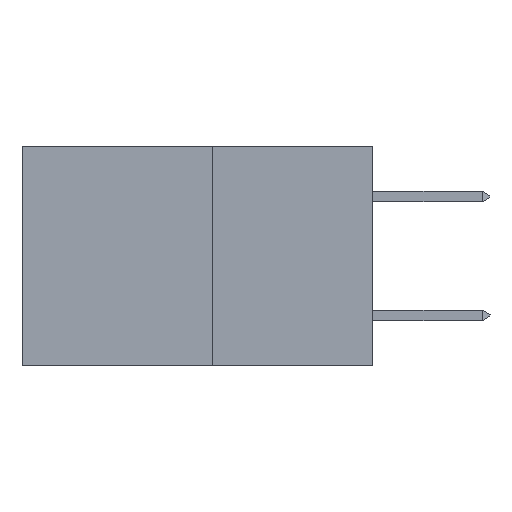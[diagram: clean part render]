
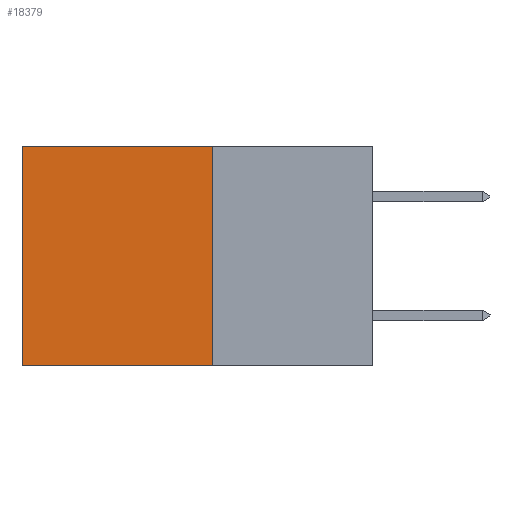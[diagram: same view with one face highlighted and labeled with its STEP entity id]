
A CAD part, left-side view. The second image highlights one B-rep face of the part: STEP entity #18379.
In plain terms, the highlighted planar face has unit normal (-1, 0, 0).
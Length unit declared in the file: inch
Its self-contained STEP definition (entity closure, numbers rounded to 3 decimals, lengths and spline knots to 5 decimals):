
#233 = DIRECTION ( 'NONE',  ( 1., 0., 0. ) ) ;
#686 = VERTEX_POINT ( 'NONE', #6723 ) ;
#3640 = LINE ( 'NONE', #4899, #29904 ) ;
#4538 = ORIENTED_EDGE ( 'NONE', *, *, #29152, .T. ) ;
#4899 = CARTESIAN_POINT ( 'NONE',  ( 0.277, 0.27, 0. ) ) ;
#6723 = CARTESIAN_POINT ( 'NONE',  ( 0.277, 0.27, -0.37 ) ) ;
#6804 = VECTOR ( 'NONE', #27416, 39.37008 ) ;
#7364 = EDGE_CURVE ( 'NONE', #28940, #26474, #14436, .T. ) ;
#8248 = VERTEX_POINT ( 'NONE', #15528 ) ;
#8363 = LINE ( 'NONE', #29169, #28668 ) ;
#8974 = ORIENTED_EDGE ( 'NONE', *, *, #29525, .F. ) ;
#9859 = DIRECTION ( 'NONE',  ( 0., 1., 0. ) ) ;
#9907 = AXIS2_PLACEMENT_3D ( 'NONE', #30683, #233, #18112 ) ;
#10705 = EDGE_LOOP ( 'NONE', ( #27272, #8974, #27764, #4538 ) ) ;
#13001 = PLANE ( 'NONE',  #9907 ) ;
#14219 = CARTESIAN_POINT ( 'NONE',  ( 0.277, 0.27, -0.37 ) ) ;
#14436 = LINE ( 'NONE', #27476, #6804 ) ;
#15528 = CARTESIAN_POINT ( 'NONE',  ( 0.277, 0.27, 0. ) ) ;
#16556 = DIRECTION ( 'NONE',  ( 0., 0., -1. ) ) ;
#17216 = LINE ( 'NONE', #14219, #30656 ) ;
#18112 = DIRECTION ( 'NONE',  ( 0., 0., -1. ) ) ;
#18379 = ADVANCED_FACE ( 'NONE', ( #25448 ), #13001, .F. ) ;
#25448 = FACE_OUTER_BOUND ( 'NONE', #10705, .T. ) ;
#26474 = VERTEX_POINT ( 'NONE', #27341 ) ;
#27115 = CARTESIAN_POINT ( 'NONE',  ( 0.277, 0.59, 0. ) ) ;
#27272 = ORIENTED_EDGE ( 'NONE', *, *, #7364, .T. ) ;
#27341 = CARTESIAN_POINT ( 'NONE',  ( 0.277, 0.59, -0.37 ) ) ;
#27416 = DIRECTION ( 'NONE',  ( 0., 0., -1. ) ) ;
#27476 = CARTESIAN_POINT ( 'NONE',  ( 0.277, 0.59, -0.37 ) ) ;
#27764 = ORIENTED_EDGE ( 'NONE', *, *, #30266, .F. ) ;
#28668 = VECTOR ( 'NONE', #16556, 39.37008 ) ;
#28940 = VERTEX_POINT ( 'NONE', #27115 ) ;
#29152 = EDGE_CURVE ( 'NONE', #8248, #28940, #3640, .T. ) ;
#29169 = CARTESIAN_POINT ( 'NONE',  ( 0.277, 0.27, -0.37 ) ) ;
#29525 = EDGE_CURVE ( 'NONE', #686, #26474, #17216, .T. ) ;
#29904 = VECTOR ( 'NONE', #9859, 39.37008 ) ;
#30266 = EDGE_CURVE ( 'NONE', #8248, #686, #8363, .T. ) ;
#30656 = VECTOR ( 'NONE', #31853, 39.37008 ) ;
#30683 = CARTESIAN_POINT ( 'NONE',  ( 0.277, 0.27, -0.37 ) ) ;
#31853 = DIRECTION ( 'NONE',  ( 0., 1., 0. ) ) ;
